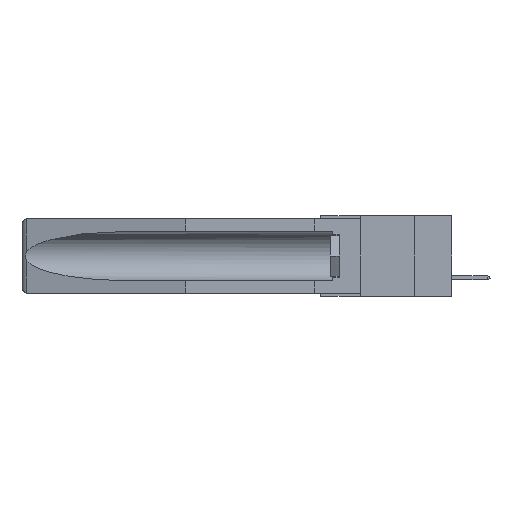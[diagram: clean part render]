
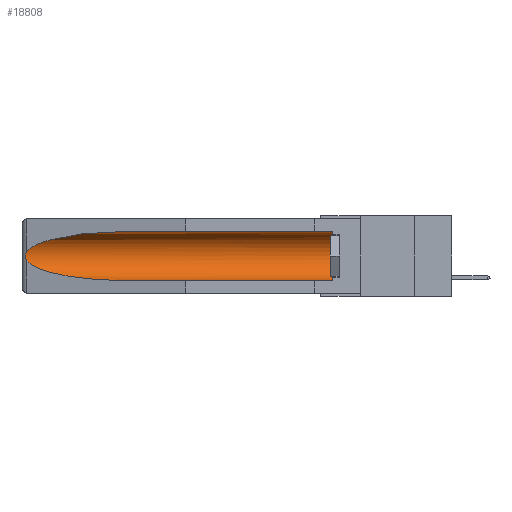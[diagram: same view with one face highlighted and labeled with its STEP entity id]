
A CAD part, left-side view. The second image highlights one B-rep face of the part: STEP entity #18808.
In plain terms, the highlighted cylindrical face has radius 2.857 mm (diameter 5.715 mm), a partial arc.
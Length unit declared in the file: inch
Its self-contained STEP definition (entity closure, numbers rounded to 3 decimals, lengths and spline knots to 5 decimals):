
#1828 = VERTEX_POINT ( 'NONE', #13678 ) ;
#1935 = CARTESIAN_POINT ( 'NONE',  ( 0.26597, 1.52961, -0.15275 ) ) ;
#2083 = CARTESIAN_POINT ( 'NONE',  ( 0.26537, 1.52718, -0.19328 ) ) ;
#2476 = CARTESIAN_POINT ( 'NONE',  ( 0.155, 0.126, -0.284 ) ) ;
#2953 = CARTESIAN_POINT ( 'NONE',  ( 0.155, 1.07973, -0.284 ) ) ;
#3339 = EDGE_CURVE ( 'NONE', #19786, #14375, #15752, .T. ) ;
#3356 = LINE ( 'NONE', #13560, #5969 ) ;
#3368 = EDGE_CURVE ( 'NONE', #7155, #19786, #8449, .T. ) ;
#3624 = CARTESIAN_POINT ( 'NONE',  ( 0.26654, 1.53092, -0.15636 ) ) ;
#3919 = CARTESIAN_POINT ( 'NONE',  ( 0.25451, 1.48313, -0.09465 ) ) ;
#4118 = CARTESIAN_POINT ( 'NONE',  ( 0.21114, 1.30732, -0.059 ) ) ;
#4490 = ORIENTED_EDGE ( 'NONE', *, *, #10191, .F. ) ;
#4667 = ORIENTED_EDGE ( 'NONE', *, *, #3339, .T. ) ;
#4885 = VERTEX_POINT ( 'NONE', #6873 ) ;
#5211 = CARTESIAN_POINT ( 'NONE',  ( 0.2673, 1.5327, -0.16383 ) ) ;
#5969 = VECTOR ( 'NONE', #11810, 39.37008 ) ;
#6707 = DIRECTION ( 'NONE',  ( 0., 0., 1. ) ) ;
#6873 = CARTESIAN_POINT ( 'NONE',  ( 0.155, 1.07973, -0.284 ) ) ;
#6901 = CARTESIAN_POINT ( 'NONE',  ( 0.26597, 1.5296, -0.19026 ) ) ;
#7155 = VERTEX_POINT ( 'NONE', #2476 ) ;
#7213 = ORIENTED_EDGE ( 'NONE', *, *, #15965, .T. ) ;
#7806 = DIRECTION ( 'NONE',  ( 0., 0., 1. ) ) ;
#7946 = DIRECTION ( 'NONE',  ( 0., 1., 0. ) ) ;
#8209 = ORIENTED_EDGE ( 'NONE', *, *, #3368, .T. ) ;
#8449 = CIRCLE ( 'NONE', #15601, 0.1125 ) ;
#8692 = CARTESIAN_POINT ( 'NONE',  ( 0.26537, 1.52718, -0.14972 ) ) ;
#9075 = EDGE_CURVE ( 'NONE', #14375, #15604, #10535, .T. ) ;
#9395 = CARTESIAN_POINT ( 'NONE',  ( 0.155, -0.30754, -0.1715 ) ) ;
#9827 =( BOUNDED_CURVE ( )  B_SPLINE_CURVE ( 3, ( #13188, #16110, #14784, #2953 ),
 .UNSPECIFIED., .F., .F. ) 
 B_SPLINE_CURVE_WITH_KNOTS ( ( 4, 4 ),
 ( 0.1948, 1.5708 ),
 .UNSPECIFIED. ) 
 CURVE ( )  GEOMETRIC_REPRESENTATION_ITEM ( )  RATIONAL_B_SPLINE_CURVE ( ( 1., 0.848, 0.848, 1. ) ) 
 REPRESENTATION_ITEM ( '' )  );
#9993 = CARTESIAN_POINT ( 'NONE',  ( 0.155, -0.30754, -0.059 ) ) ;
#10191 = EDGE_CURVE ( 'NONE', #7155, #4885, #3356, .T. ) ;
#10252 = DIRECTION ( 'NONE',  ( 0., 1., 0. ) ) ;
#10428 = CARTESIAN_POINT ( 'NONE',  ( 0.2675, 1.53308, -0.17534 ) ) ;
#10535 =( BOUNDED_CURVE ( )  B_SPLINE_CURVE ( 3, ( #19019, #4118, #3919, #14060 ),
 .UNSPECIFIED., .F., .F. ) 
 B_SPLINE_CURVE_WITH_KNOTS ( ( 4, 4 ),
 ( 4.71239, 6.08839 ),
 .UNSPECIFIED. ) 
 CURVE ( )  GEOMETRIC_REPRESENTATION_ITEM ( )  RATIONAL_B_SPLINE_CURVE ( ( 1., 0.848, 0.848, 1. ) ) 
 REPRESENTATION_ITEM ( '' )  );
#11049 = VECTOR ( 'NONE', #10252, 39.37008 ) ;
#11810 = DIRECTION ( 'NONE',  ( 0., 1., 0. ) ) ;
#12103 = CARTESIAN_POINT ( 'NONE',  ( 0.2673, 1.53269, -0.17917 ) ) ;
#12577 = ORIENTED_EDGE ( 'NONE', *, *, #16998, .T. ) ;
#12734 = ORIENTED_EDGE ( 'NONE', *, *, #9075, .T. ) ;
#12794 = B_SPLINE_CURVE_WITH_KNOTS ( 'NONE', 3,
 ( #8692, #1935, #3624, #5211, #17052, #10428, #12103, #15459, #6901, #2083 ),
 .UNSPECIFIED., .F., .F.,
 ( 4, 2, 2, 2, 4 ),
 ( 0., 0.00029, 0.00058, 0.00087, 0.00117 ),
 .UNSPECIFIED. ) ;
#13188 = CARTESIAN_POINT ( 'NONE',  ( 0.26537, 1.52718, -0.19328 ) ) ;
#13496 = CARTESIAN_POINT ( 'NONE',  ( 0.155, 0.126, -0.059 ) ) ;
#13560 = CARTESIAN_POINT ( 'NONE',  ( 0.155, -0.30754, -0.284 ) ) ;
#13678 = CARTESIAN_POINT ( 'NONE',  ( 0.26537, 1.52718, -0.19328 ) ) ;
#14060 = CARTESIAN_POINT ( 'NONE',  ( 0.26537, 1.52718, -0.14972 ) ) ;
#14375 = VERTEX_POINT ( 'NONE', #17889 ) ;
#14763 = CARTESIAN_POINT ( 'NONE',  ( 0.26537, 1.52718, -0.14972 ) ) ;
#14784 = CARTESIAN_POINT ( 'NONE',  ( 0.21114, 1.30732, -0.284 ) ) ;
#15459 = CARTESIAN_POINT ( 'NONE',  ( 0.26655, 1.53094, -0.18657 ) ) ;
#15601 = AXIS2_PLACEMENT_3D ( 'NONE', #16703, #18314, #6707 ) ;
#15604 = VERTEX_POINT ( 'NONE', #14763 ) ;
#15752 = LINE ( 'NONE', #9993, #11049 ) ;
#15965 = EDGE_CURVE ( 'NONE', #1828, #4885, #9827, .T. ) ;
#16104 = EDGE_LOOP ( 'NONE', ( #12734, #12577, #7213, #4490, #8209, #4667 ) ) ;
#16110 = CARTESIAN_POINT ( 'NONE',  ( 0.25451, 1.48313, -0.24835 ) ) ;
#16703 = CARTESIAN_POINT ( 'NONE',  ( 0.155, 0.126, -0.1715 ) ) ;
#16998 = EDGE_CURVE ( 'NONE', #15604, #1828, #12794, .T. ) ;
#17052 = CARTESIAN_POINT ( 'NONE',  ( 0.2675, 1.53308, -0.16763 ) ) ;
#17889 = CARTESIAN_POINT ( 'NONE',  ( 0.155, 1.07973, -0.059 ) ) ;
#18314 = DIRECTION ( 'NONE',  ( 0., -1., 0. ) ) ;
#18808 = ADVANCED_FACE ( 'NONE', ( #21104 ), #20081, .F. ) ;
#19019 = CARTESIAN_POINT ( 'NONE',  ( 0.155, 1.07973, -0.059 ) ) ;
#19786 = VERTEX_POINT ( 'NONE', #13496 ) ;
#20081 = CYLINDRICAL_SURFACE ( 'NONE', #20649, 0.1125 ) ;
#20649 = AXIS2_PLACEMENT_3D ( 'NONE', #9395, #7946, #7806 ) ;
#21104 = FACE_OUTER_BOUND ( 'NONE', #16104, .T. ) ;
